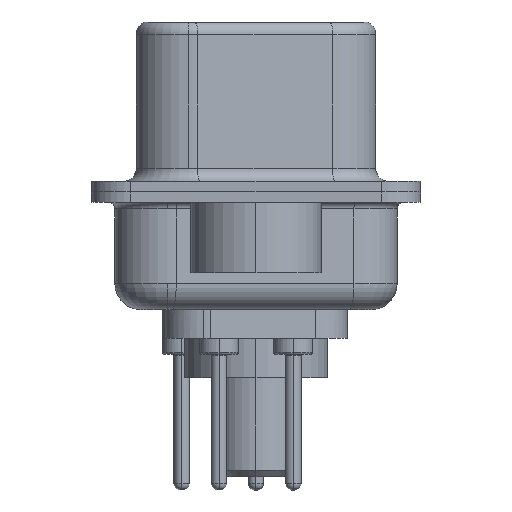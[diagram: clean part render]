
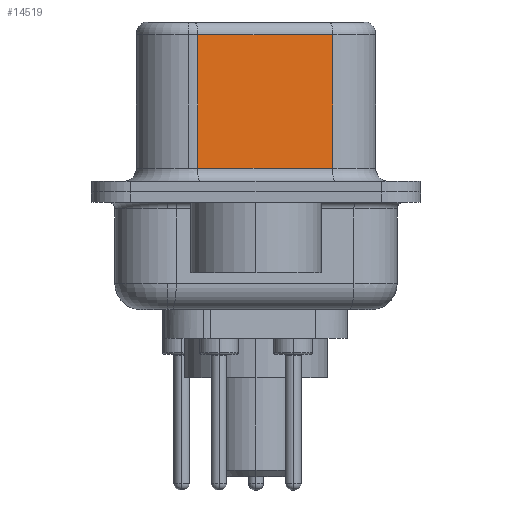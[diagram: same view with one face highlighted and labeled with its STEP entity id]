
A CAD part, left-side view. The second image highlights one B-rep face of the part: STEP entity #14519.
In plain terms, the highlighted planar face has unit normal (-0.985, -0.174, 0).
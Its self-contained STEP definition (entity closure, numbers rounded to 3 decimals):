
#292 = LINE ( 'NONE', #13188, #22191 ) ;
#587 = EDGE_CURVE ( 'NONE', #6684, #19734, #292, .T. ) ;
#937 = AXIS2_PLACEMENT_3D ( 'NONE', #14293, #23159, #16039 ) ;
#2537 = CARTESIAN_POINT ( 'NONE',  ( 3.675, 2.233, 6.52 ) ) ;
#2908 = CARTESIAN_POINT ( 'NONE',  ( 4.585, -2.927, 6.02 ) ) ;
#3093 = CARTESIAN_POINT ( 'NONE',  ( 4.585, -2.927, 0.9 ) ) ;
#4747 = CARTESIAN_POINT ( 'NONE',  ( 3.675, 2.233, 6.02 ) ) ;
#5897 = DIRECTION ( 'NONE',  ( 0.174, -0.985, 0. ) ) ;
#6426 = EDGE_CURVE ( 'NONE', #14242, #19734, #8239, .T. ) ;
#6684 = VERTEX_POINT ( 'NONE', #7224 ) ;
#7224 = CARTESIAN_POINT ( 'NONE',  ( 4.585, -2.927, 6.02 ) ) ;
#7823 = ORIENTED_EDGE ( 'NONE', *, *, #6426, .T. ) ;
#7844 = FACE_OUTER_BOUND ( 'NONE', #19363, .T. ) ;
#8169 = ORIENTED_EDGE ( 'NONE', *, *, #9973, .T. ) ;
#8191 = DIRECTION ( 'NONE',  ( 0., 0., -1. ) ) ;
#8239 = LINE ( 'NONE', #20095, #13828 ) ;
#8531 = ORIENTED_EDGE ( 'NONE', *, *, #587, .F. ) ;
#9770 = VECTOR ( 'NONE', #11748, 1000. ) ;
#9973 = EDGE_CURVE ( 'NONE', #12348, #14242, #13604, .T. ) ;
#11446 = LINE ( 'NONE', #2908, #9770 ) ;
#11565 = ORIENTED_EDGE ( 'NONE', *, *, #22459, .T. ) ;
#11748 = DIRECTION ( 'NONE',  ( -0.174, 0.985, 0. ) ) ;
#12348 = VERTEX_POINT ( 'NONE', #4747 ) ;
#13188 = CARTESIAN_POINT ( 'NONE',  ( 4.585, -2.927, 6.52 ) ) ;
#13604 = LINE ( 'NONE', #2537, #16987 ) ;
#13828 = VECTOR ( 'NONE', #5897, 1000. ) ;
#14213 = PLANE ( 'NONE',  #937 ) ;
#14242 = VERTEX_POINT ( 'NONE', #21557 ) ;
#14293 = CARTESIAN_POINT ( 'NONE',  ( 4.585, -2.927, 6.52 ) ) ;
#14519 = ADVANCED_FACE ( 'NONE', ( #7844 ), #14213, .F. ) ;
#15024 = DIRECTION ( 'NONE',  ( 0., 0., -1. ) ) ;
#16039 = DIRECTION ( 'NONE',  ( -0.174, 0.985, 0. ) ) ;
#16987 = VECTOR ( 'NONE', #8191, 1000. ) ;
#19363 = EDGE_LOOP ( 'NONE', ( #8531, #11565, #8169, #7823 ) ) ;
#19734 = VERTEX_POINT ( 'NONE', #3093 ) ;
#20095 = CARTESIAN_POINT ( 'NONE',  ( 4.585, -2.927, 0.9 ) ) ;
#21557 = CARTESIAN_POINT ( 'NONE',  ( 3.675, 2.233, 0.9 ) ) ;
#22191 = VECTOR ( 'NONE', #15024, 1000. ) ;
#22459 = EDGE_CURVE ( 'NONE', #6684, #12348, #11446, .T. ) ;
#23159 = DIRECTION ( 'NONE',  ( 0.985, 0.174, 0. ) ) ;
